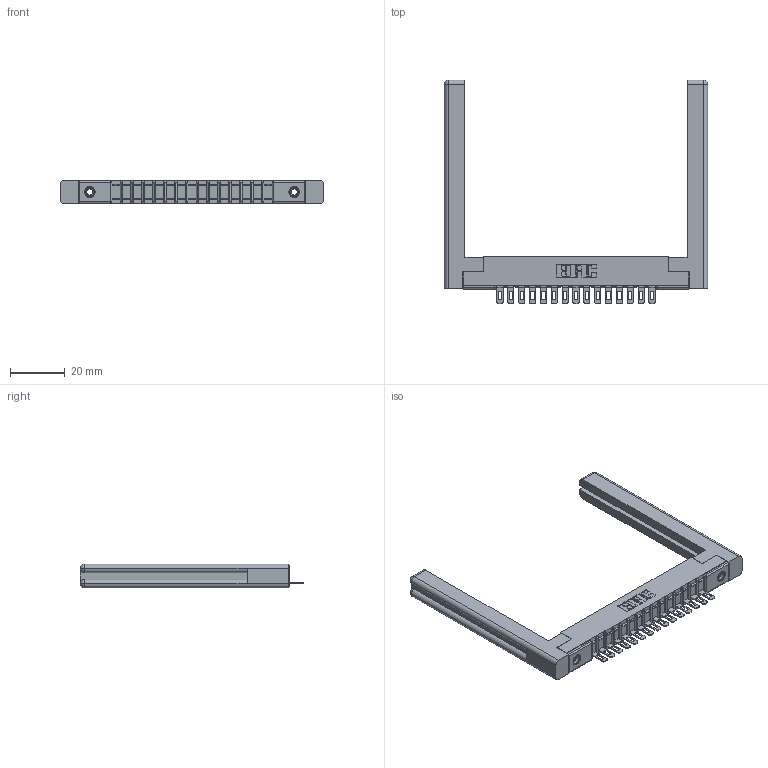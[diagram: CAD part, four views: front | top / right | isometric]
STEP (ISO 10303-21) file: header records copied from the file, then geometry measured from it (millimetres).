
FILE_DESCRIPTION (( 'STEP AP203' ), '1' );
FILE_NAME ('307-015-401-158.STEP', '2020-09-25T17:34:37', ( '' ), ( '' ), 'SwSTEP 2.0', 'SolidWorks 2020', '' );
FILE_SCHEMA (( 'CONFIG_CONTROL_DESIGN' ));
Length unit declared in the file: inch
Products named in the file (5): 345-250-001_345-250-001-102; 307 Part_.156 Dia Mounting Holes; 307-015-401-158; 307-220-058; 307-290-002_501
Assembly tree (20 placements, depth 2):
  307-015-401-158
    307 Part_.156 Dia Mounting Holes
    307-290-002_501  x15
    307-220-058  x2
    345-250-001_345-250-001-102  x2
Bounding box: 96.06 x 81.74 x 8.71 mm (x, y, z)
Volume: 14029.6 mm3; surface area: 16288 mm2
Topology: 20 solids, 20 shells, 1416 faces, 4247 edges, 2774 vertices
Faces by surface type: plane 814, cylinder 546, sphere 32, torus 12, cone 12
Entity records: 19615 total; most frequent: CARTESIAN_POINT 3311, ORIENTED_EDGE 3240, DIRECTION 3194, EDGE_CURVE 1620, LINE 1220, VECTOR 1220, VERTEX_POINT 1050, AXIS2_PLACEMENT_3D 987
